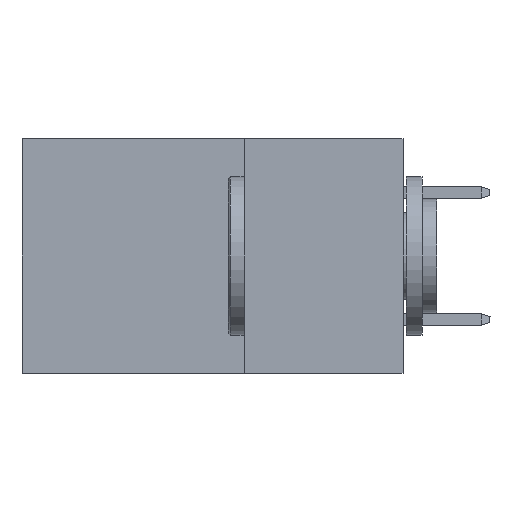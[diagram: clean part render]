
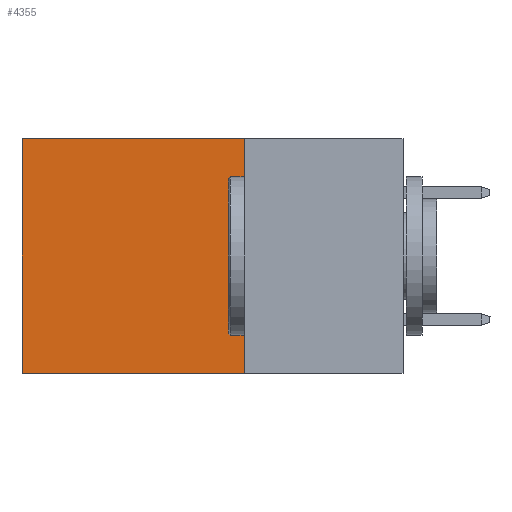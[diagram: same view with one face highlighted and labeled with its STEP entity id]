
A CAD part, left-side view. The second image highlights one B-rep face of the part: STEP entity #4355.
In plain terms, the highlighted planar face has unit normal (-1, 0, 0).
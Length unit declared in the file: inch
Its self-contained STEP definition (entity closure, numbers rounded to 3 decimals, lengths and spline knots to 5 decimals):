
#286 = PLANE ( 'NONE',  #7084 ) ;
#676 = LINE ( 'NONE', #1833, #12881 ) ;
#1211 = EDGE_LOOP ( 'NONE', ( #13021, #4543, #13594, #11794 ) ) ;
#1728 = CARTESIAN_POINT ( 'NONE',  ( 0.2875, 0.25, 0. ) ) ;
#1833 = CARTESIAN_POINT ( 'NONE',  ( 0.2875, 0.25, -0.37 ) ) ;
#1983 = CARTESIAN_POINT ( 'NONE',  ( 0.2875, 0.25, -0.37 ) ) ;
#3172 = VERTEX_POINT ( 'NONE', #7967 ) ;
#3595 = VERTEX_POINT ( 'NONE', #1983 ) ;
#3977 = VERTEX_POINT ( 'NONE', #4315 ) ;
#4264 = LINE ( 'NONE', #7297, #8693 ) ;
#4315 = CARTESIAN_POINT ( 'NONE',  ( 0.2875, 0.25, 0. ) ) ;
#4355 = ADVANCED_FACE ( 'NONE', ( #17932 ), #286, .F. ) ;
#4543 = ORIENTED_EDGE ( 'NONE', *, *, #12635, .F. ) ;
#4750 = DIRECTION ( 'NONE',  ( 1., 0., 0. ) ) ;
#6483 = CARTESIAN_POINT ( 'NONE',  ( 0.2875, 0.25, 0. ) ) ;
#7084 = AXIS2_PLACEMENT_3D ( 'NONE', #1728, #4750, #10510 ) ;
#7113 = DIRECTION ( 'NONE',  ( 0., 1., 0. ) ) ;
#7297 = CARTESIAN_POINT ( 'NONE',  ( 0.2875, 0.25, 0. ) ) ;
#7446 = VERTEX_POINT ( 'NONE', #18537 ) ;
#7724 = EDGE_CURVE ( 'NONE', #3977, #3595, #14044, .T. ) ;
#7796 = DIRECTION ( 'NONE',  ( 0., 1., 0. ) ) ;
#7967 = CARTESIAN_POINT ( 'NONE',  ( 0.2875, 0.6, 0. ) ) ;
#8181 = DIRECTION ( 'NONE',  ( 0., 0., -1. ) ) ;
#8320 = VECTOR ( 'NONE', #17206, 39.37008 ) ;
#8693 = VECTOR ( 'NONE', #7113, 39.37008 ) ;
#10414 = EDGE_CURVE ( 'NONE', #3172, #7446, #15773, .T. ) ;
#10510 = DIRECTION ( 'NONE',  ( 0., 0., -1. ) ) ;
#11277 = VECTOR ( 'NONE', #8181, 39.37008 ) ;
#11382 = CARTESIAN_POINT ( 'NONE',  ( 0.2875, 0.6, 0. ) ) ;
#11794 = ORIENTED_EDGE ( 'NONE', *, *, #14197, .T. ) ;
#12635 = EDGE_CURVE ( 'NONE', #3595, #7446, #676, .T. ) ;
#12881 = VECTOR ( 'NONE', #7796, 39.37008 ) ;
#13021 = ORIENTED_EDGE ( 'NONE', *, *, #10414, .T. ) ;
#13594 = ORIENTED_EDGE ( 'NONE', *, *, #7724, .F. ) ;
#14044 = LINE ( 'NONE', #6483, #11277 ) ;
#14197 = EDGE_CURVE ( 'NONE', #3977, #3172, #4264, .T. ) ;
#15773 = LINE ( 'NONE', #11382, #8320 ) ;
#17206 = DIRECTION ( 'NONE',  ( 0., 0., -1. ) ) ;
#17932 = FACE_OUTER_BOUND ( 'NONE', #1211, .T. ) ;
#18537 = CARTESIAN_POINT ( 'NONE',  ( 0.2875, 0.6, -0.37 ) ) ;
